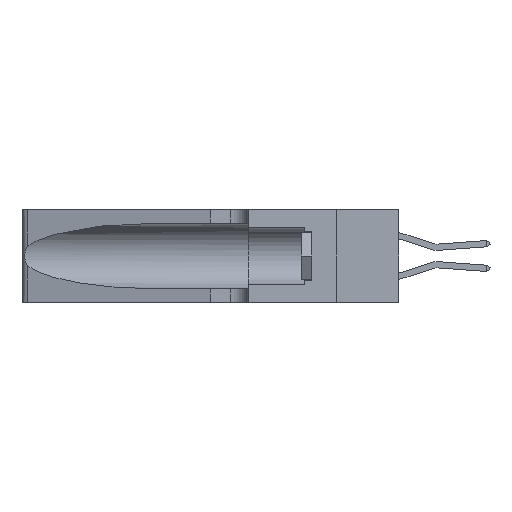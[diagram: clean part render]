
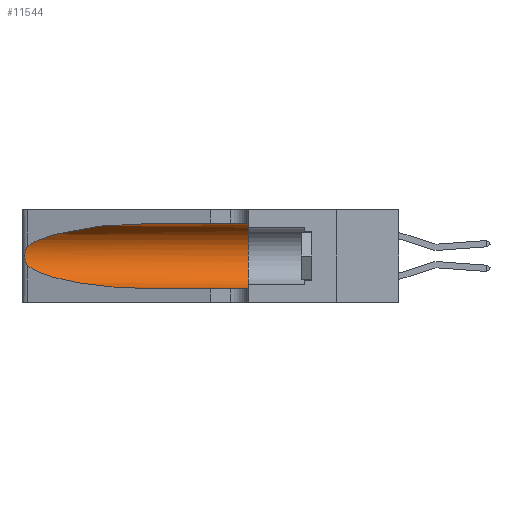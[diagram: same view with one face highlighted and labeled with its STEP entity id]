
A CAD part, left-side view. The second image highlights one B-rep face of the part: STEP entity #11544.
In plain terms, the highlighted cylindrical face has radius 3.308 mm (diameter 6.617 mm), a partial arc.
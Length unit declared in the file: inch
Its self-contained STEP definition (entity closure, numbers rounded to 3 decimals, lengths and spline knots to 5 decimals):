
#839 = DIRECTION ( 'NONE',  ( 0., -1., 0. ) ) ;
#1109 = CARTESIAN_POINT ( 'NONE',  ( 0.26075, 1.23896, 0.178 ) ) ;
#1181 = CARTESIAN_POINT ( 'NONE',  ( 0.25487, 1.22718, 0.14631 ) ) ;
#1753 = CARTESIAN_POINT ( 'NONE',  ( 0.1305, 1.61858, 0.05475 ) ) ;
#2022 = CARTESIAN_POINT ( 'NONE',  ( 0.1305, 0.72297, 0.31525 ) ) ;
#2138 = VECTOR ( 'NONE', #9804, 39.37008 ) ;
#2498 = VERTEX_POINT ( 'NONE', #13582 ) ;
#2585 = AXIS2_PLACEMENT_3D ( 'NONE', #18693, #839, #6996 ) ;
#3166 = CARTESIAN_POINT ( 'NONE',  ( 0.25856, 1.23593, 0.16098 ) ) ;
#3270 = ORIENTED_EDGE ( 'NONE', *, *, #7021, .T. ) ;
#3541 = ORIENTED_EDGE ( 'NONE', *, *, #21524, .T. ) ;
#3812 = DIRECTION ( 'NONE',  ( 0., -1., 0. ) ) ;
#4222 = ORIENTED_EDGE ( 'NONE', *, *, #24057, .T. ) ;
#4248 = ORIENTED_EDGE ( 'NONE', *, *, #15076, .T. ) ;
#4456 = VERTEX_POINT ( 'NONE', #11855 ) ;
#4582 =( BOUNDED_CURVE ( )  B_SPLINE_CURVE ( 3, ( #2022, #13967, #9967, #15911 ),
 .UNSPECIFIED., .F., .F. ) 
 B_SPLINE_CURVE_WITH_KNOTS ( ( 4, 4 ),
 ( 1.5708, 2.84003 ),
 .UNSPECIFIED. ) 
 CURVE ( )  GEOMETRIC_REPRESENTATION_ITEM ( )  RATIONAL_B_SPLINE_CURVE ( ( 1., 0.87, 0.87, 1. ) ) 
 REPRESENTATION_ITEM ( '' )  );
#4778 = VECTOR ( 'NONE', #3812, 39.37008 ) ;
#4824 = ORIENTED_EDGE ( 'NONE', *, *, #16705, .F. ) ;
#4876 = ORIENTED_EDGE ( 'NONE', *, *, #11172, .F. ) ;
#4991 = VERTEX_POINT ( 'NONE', #15410 ) ;
#5230 = CARTESIAN_POINT ( 'NONE',  ( 0.25639, 1.23186, 0.15144 ) ) ;
#5311 = CARTESIAN_POINT ( 'NONE',  ( 0.1305, 0.72297, 0.05475 ) ) ;
#6422 = AXIS2_PLACEMENT_3D ( 'NONE', #21766, #10200, #23676 ) ;
#6996 = DIRECTION ( 'NONE',  ( 0., 0., -1. ) ) ;
#7021 = EDGE_CURVE ( 'NONE', #8705, #21067, #4582, .T. ) ;
#7252 = CARTESIAN_POINT ( 'NONE',  ( 0.25487, 1.22718, 0.14631 ) ) ;
#7547 = LINE ( 'NONE', #7804, #2138 ) ;
#7804 = CARTESIAN_POINT ( 'NONE',  ( 0.1305, 1.61858, 0.31525 ) ) ;
#8132 = FACE_OUTER_BOUND ( 'NONE', #11056, .T. ) ;
#8705 = VERTEX_POINT ( 'NONE', #18379 ) ;
#9152 = CARTESIAN_POINT ( 'NONE',  ( 0.25639, 1.23184, 0.21858 ) ) ;
#9804 = DIRECTION ( 'NONE',  ( 0., -1., 0. ) ) ;
#9967 = CARTESIAN_POINT ( 'NONE',  ( 0.2373, 1.15595, 0.28018 ) ) ;
#10200 = DIRECTION ( 'NONE',  ( 0., 1., 0. ) ) ;
#10655 = CARTESIAN_POINT ( 'NONE',  ( 0.1305, 0.35, 0.05475 ) ) ;
#10907 = VERTEX_POINT ( 'NONE', #10655 ) ;
#11056 = EDGE_LOOP ( 'NONE', ( #3270, #3541, #4222, #4248, #4824, #4876 ) ) ;
#11149 = CARTESIAN_POINT ( 'NONE',  ( 0.25854, 1.2359, 0.20912 ) ) ;
#11172 = EDGE_CURVE ( 'NONE', #8705, #2498, #7547, .T. ) ;
#11488 = CIRCLE ( 'NONE', #6422, 0.13025 ) ;
#11544 = ADVANCED_FACE ( 'NONE', ( #8132 ), #22988, .F. ) ;
#11855 = CARTESIAN_POINT ( 'NONE',  ( 0.1305, 0.72297, 0.05475 ) ) ;
#11908 = B_SPLINE_CURVE_WITH_KNOTS ( 'NONE', 3,
 ( #16910, #14971, #9152, #22692, #11149, #24600, #13107, #1109, #15053, #3166, #16993, #5230, #18922, #7252 ),
 .UNSPECIFIED., .F., .F.,
 ( 4, 2, 2, 2, 2, 2, 4 ),
 ( 0., 0.00027, 0.00053, 0.00107, 0.0016, 0.00187, 0.00214 ),
 .UNSPECIFIED. ) ;
#13107 = CARTESIAN_POINT ( 'NONE',  ( 0.26075, 1.23896, 0.19203 ) ) ;
#13182 = CARTESIAN_POINT ( 'NONE',  ( 0.2373, 1.15595, 0.08982 ) ) ;
#13582 = CARTESIAN_POINT ( 'NONE',  ( 0.1305, 0.35, 0.31525 ) ) ;
#13967 = CARTESIAN_POINT ( 'NONE',  ( 0.18966, 0.96281, 0.31525 ) ) ;
#14971 = CARTESIAN_POINT ( 'NONE',  ( 0.25555, 1.22994, 0.2215 ) ) ;
#15053 = CARTESIAN_POINT ( 'NONE',  ( 0.26017, 1.23833, 0.17102 ) ) ;
#15076 = EDGE_CURVE ( 'NONE', #4456, #10907, #24460, .T. ) ;
#15410 = CARTESIAN_POINT ( 'NONE',  ( 0.25487, 1.22718, 0.14631 ) ) ;
#15911 = CARTESIAN_POINT ( 'NONE',  ( 0.25487, 1.22718, 0.22369 ) ) ;
#16705 = EDGE_CURVE ( 'NONE', #2498, #10907, #11488, .T. ) ;
#16910 = CARTESIAN_POINT ( 'NONE',  ( 0.25487, 1.22718, 0.22369 ) ) ;
#16993 = CARTESIAN_POINT ( 'NONE',  ( 0.25789, 1.23486, 0.15765 ) ) ;
#17062 = CARTESIAN_POINT ( 'NONE',  ( 0.18966, 0.96281, 0.05475 ) ) ;
#18379 = CARTESIAN_POINT ( 'NONE',  ( 0.1305, 0.72297, 0.31525 ) ) ;
#18693 = CARTESIAN_POINT ( 'NONE',  ( 0.1305, 1.61858, 0.185 ) ) ;
#18922 = CARTESIAN_POINT ( 'NONE',  ( 0.25555, 1.22993, 0.14849 ) ) ;
#21067 = VERTEX_POINT ( 'NONE', #23128 ) ;
#21524 = EDGE_CURVE ( 'NONE', #21067, #4991, #11908, .T. ) ;
#21766 = CARTESIAN_POINT ( 'NONE',  ( 0.1305, 0.35, 0.185 ) ) ;
#22692 = CARTESIAN_POINT ( 'NONE',  ( 0.25787, 1.23484, 0.2124 ) ) ;
#22988 = CYLINDRICAL_SURFACE ( 'NONE', #2585, 0.13025 ) ;
#23128 = CARTESIAN_POINT ( 'NONE',  ( 0.25487, 1.22718, 0.22369 ) ) ;
#23486 =( BOUNDED_CURVE ( )  B_SPLINE_CURVE ( 3, ( #1181, #13182, #17062, #5311 ),
 .UNSPECIFIED., .F., .T. ) 
 B_SPLINE_CURVE_WITH_KNOTS ( ( 4, 4 ),
 ( 3.44316, 4.71239 ),
 .UNSPECIFIED. ) 
 CURVE ( )  GEOMETRIC_REPRESENTATION_ITEM ( )  RATIONAL_B_SPLINE_CURVE ( ( 1., 0.87, 0.87, 1. ) ) 
 REPRESENTATION_ITEM ( '' )  );
#23676 = DIRECTION ( 'NONE',  ( 0., 0., 1. ) ) ;
#24057 = EDGE_CURVE ( 'NONE', #4991, #4456, #23486, .T. ) ;
#24460 = LINE ( 'NONE', #1753, #4778 ) ;
#24600 = CARTESIAN_POINT ( 'NONE',  ( 0.26018, 1.23835, 0.19895 ) ) ;
